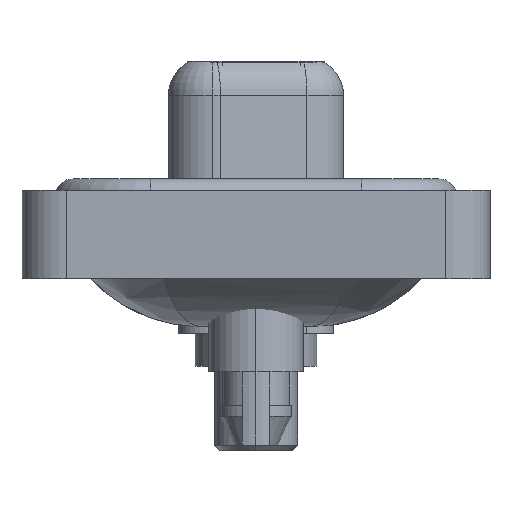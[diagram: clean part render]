
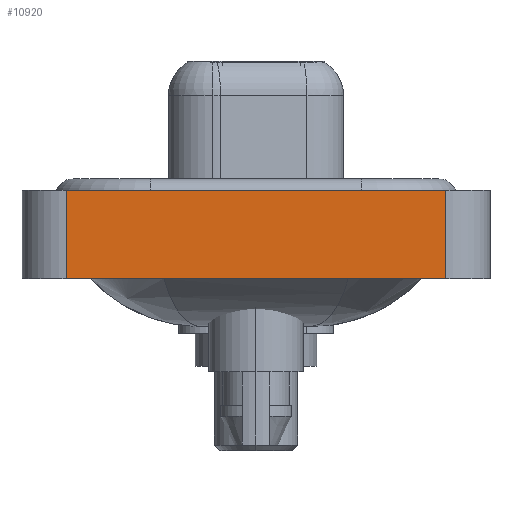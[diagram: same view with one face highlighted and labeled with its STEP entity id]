
A CAD part, left-side view. The second image highlights one B-rep face of the part: STEP entity #10920.
In plain terms, the highlighted planar face has unit normal (-1, 0, 0).
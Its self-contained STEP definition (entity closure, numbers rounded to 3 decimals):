
#366 = VERTEX_POINT ( 'NONE', #10573 ) ;
#646 = VECTOR ( 'NONE', #12281, 1000. ) ;
#816 = VERTEX_POINT ( 'NONE', #15333 ) ;
#2122 = FACE_OUTER_BOUND ( 'NONE', #12450, .T. ) ;
#2128 = CARTESIAN_POINT ( 'NONE',  ( -7.3, -8.55, 0.4 ) ) ;
#2210 = PLANE ( 'NONE',  #12009 ) ;
#3484 = EDGE_CURVE ( 'NONE', #15318, #11829, #16575, .T. ) ;
#4833 = ORIENTED_EDGE ( 'NONE', *, *, #14578, .F. ) ;
#4846 = DIRECTION ( 'NONE',  ( 0., 0., 1. ) ) ;
#5112 = CARTESIAN_POINT ( 'NONE',  ( -7.3, 8.55, -3.6 ) ) ;
#5842 = VECTOR ( 'NONE', #7181, 1000. ) ;
#6465 = LINE ( 'NONE', #5112, #8737 ) ;
#6579 = ORIENTED_EDGE ( 'NONE', *, *, #10705, .T. ) ;
#7181 = DIRECTION ( 'NONE',  ( 0., -1., 0. ) ) ;
#7302 = CARTESIAN_POINT ( 'NONE',  ( -7.3, -8.55, -3.6 ) ) ;
#7335 = LINE ( 'NONE', #11102, #646 ) ;
#7397 = DIRECTION ( 'NONE',  ( 0., 0., 1. ) ) ;
#7464 = ORIENTED_EDGE ( 'NONE', *, *, #3484, .F. ) ;
#7674 = DIRECTION ( 'NONE',  ( 0., 0., 1. ) ) ;
#8737 = VECTOR ( 'NONE', #4846, 1000. ) ;
#9641 = EDGE_CURVE ( 'NONE', #816, #11829, #10401, .T. ) ;
#10401 = LINE ( 'NONE', #15748, #11520 ) ;
#10573 = CARTESIAN_POINT ( 'NONE',  ( -7.3, 8.55, -3.6 ) ) ;
#10705 = EDGE_CURVE ( 'NONE', #366, #816, #7335, .T. ) ;
#10920 = ADVANCED_FACE ( 'NONE', ( #2122 ), #2210, .T. ) ;
#11102 = CARTESIAN_POINT ( 'NONE',  ( -7.3, -8.55, -3.6 ) ) ;
#11520 = VECTOR ( 'NONE', #7674, 1000. ) ;
#11829 = VERTEX_POINT ( 'NONE', #2128 ) ;
#12009 = AXIS2_PLACEMENT_3D ( 'NONE', #7302, #16606, #7397 ) ;
#12281 = DIRECTION ( 'NONE',  ( 0., -1., 0. ) ) ;
#12450 = EDGE_LOOP ( 'NONE', ( #13330, #7464, #4833, #6579 ) ) ;
#12480 = CARTESIAN_POINT ( 'NONE',  ( -7.3, -8.55, 0.4 ) ) ;
#13330 = ORIENTED_EDGE ( 'NONE', *, *, #9641, .T. ) ;
#14578 = EDGE_CURVE ( 'NONE', #366, #15318, #6465, .T. ) ;
#15318 = VERTEX_POINT ( 'NONE', #15327 ) ;
#15327 = CARTESIAN_POINT ( 'NONE',  ( -7.3, 8.55, 0.4 ) ) ;
#15333 = CARTESIAN_POINT ( 'NONE',  ( -7.3, -8.55, -3.6 ) ) ;
#15748 = CARTESIAN_POINT ( 'NONE',  ( -7.3, -8.55, -3.6 ) ) ;
#16575 = LINE ( 'NONE', #12480, #5842 ) ;
#16606 = DIRECTION ( 'NONE',  ( -1., 0., 0. ) ) ;
